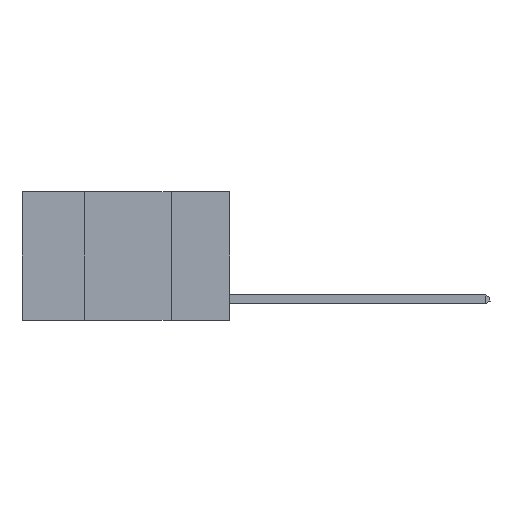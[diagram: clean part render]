
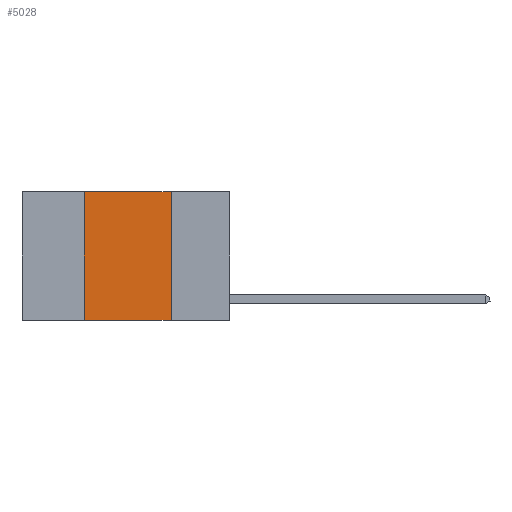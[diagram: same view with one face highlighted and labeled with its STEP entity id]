
A CAD part, left-side view. The second image highlights one B-rep face of the part: STEP entity #5028.
In plain terms, the highlighted planar face has unit normal (-1, 0, 0).
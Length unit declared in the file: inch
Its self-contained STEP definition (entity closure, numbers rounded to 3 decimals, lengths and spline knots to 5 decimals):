
#856 = DIRECTION ( 'NONE',  ( 0., -1., 0. ) ) ;
#1647 = CARTESIAN_POINT ( 'NONE',  ( 0., 0.17, -0.37 ) ) ;
#1780 = DIRECTION ( 'NONE',  ( 1., 0., 0. ) ) ;
#2072 = DIRECTION ( 'NONE',  ( 0., 0., -1. ) ) ;
#2565 = LINE ( 'NONE', #14693, #3361 ) ;
#3035 = DIRECTION ( 'NONE',  ( 0., 0., 1. ) ) ;
#3361 = VECTOR ( 'NONE', #856, 39.37008 ) ;
#3506 = EDGE_CURVE ( 'NONE', #16335, #4958, #11833, .T. ) ;
#3989 = VECTOR ( 'NONE', #8248, 39.37008 ) ;
#4707 = EDGE_CURVE ( 'NONE', #11445, #16752, #16018, .T. ) ;
#4958 = VERTEX_POINT ( 'NONE', #6038 ) ;
#5028 = ADVANCED_FACE ( 'NONE', ( #10204 ), #7317, .F. ) ;
#5600 = CARTESIAN_POINT ( 'NONE',  ( 0., 0.6, -0.37 ) ) ;
#5644 = EDGE_LOOP ( 'NONE', ( #8136, #13849, #16769, #11615 ) ) ;
#6038 = CARTESIAN_POINT ( 'NONE',  ( 0., 0.42, 0. ) ) ;
#7153 = LINE ( 'NONE', #5600, #3989 ) ;
#7317 = PLANE ( 'NONE',  #9857 ) ;
#8136 = ORIENTED_EDGE ( 'NONE', *, *, #4707, .F. ) ;
#8248 = DIRECTION ( 'NONE',  ( 0., -1., 0. ) ) ;
#9418 = CARTESIAN_POINT ( 'NONE',  ( 0., 0.17, 0. ) ) ;
#9421 = VECTOR ( 'NONE', #3035, 39.37008 ) ;
#9857 = AXIS2_PLACEMENT_3D ( 'NONE', #14358, #1780, #17002 ) ;
#9995 = CARTESIAN_POINT ( 'NONE',  ( 0., 0.42, -0.37 ) ) ;
#10204 = FACE_OUTER_BOUND ( 'NONE', #5644, .T. ) ;
#11445 = VERTEX_POINT ( 'NONE', #17722 ) ;
#11615 = ORIENTED_EDGE ( 'NONE', *, *, #15884, .T. ) ;
#11833 = LINE ( 'NONE', #14645, #9421 ) ;
#13849 = ORIENTED_EDGE ( 'NONE', *, *, #14010, .F. ) ;
#14010 = EDGE_CURVE ( 'NONE', #4958, #11445, #2565, .T. ) ;
#14358 = CARTESIAN_POINT ( 'NONE',  ( 0., 0.6, 0. ) ) ;
#14645 = CARTESIAN_POINT ( 'NONE',  ( 0., 0.42, 0. ) ) ;
#14693 = CARTESIAN_POINT ( 'NONE',  ( 0., 0.6, 0. ) ) ;
#15884 = EDGE_CURVE ( 'NONE', #16335, #16752, #7153, .T. ) ;
#16018 = LINE ( 'NONE', #9418, #16796 ) ;
#16335 = VERTEX_POINT ( 'NONE', #9995 ) ;
#16752 = VERTEX_POINT ( 'NONE', #1647 ) ;
#16769 = ORIENTED_EDGE ( 'NONE', *, *, #3506, .F. ) ;
#16796 = VECTOR ( 'NONE', #2072, 39.37008 ) ;
#17002 = DIRECTION ( 'NONE',  ( 0., 0., -1. ) ) ;
#17722 = CARTESIAN_POINT ( 'NONE',  ( 0., 0.17, 0. ) ) ;
